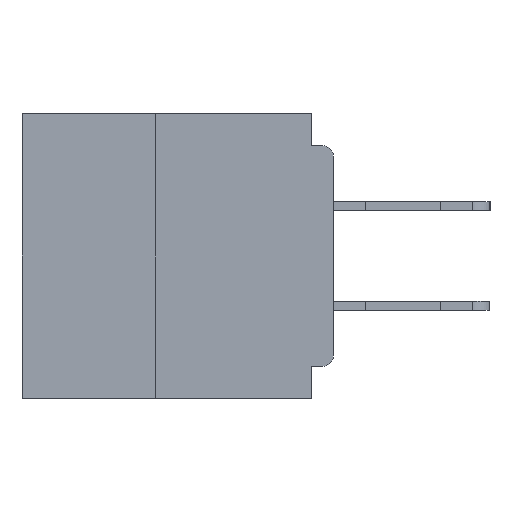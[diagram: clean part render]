
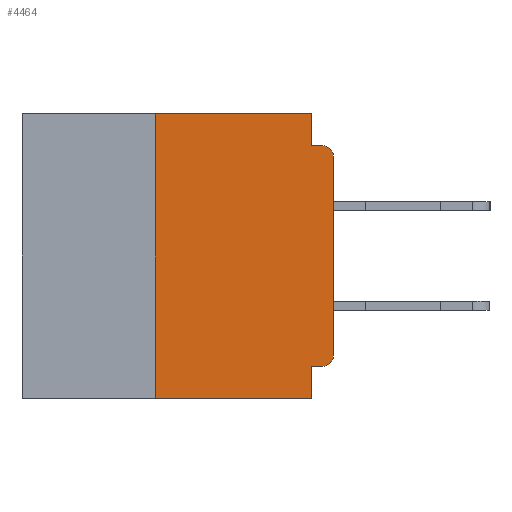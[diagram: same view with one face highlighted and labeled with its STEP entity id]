
A CAD part, left-side view. The second image highlights one B-rep face of the part: STEP entity #4464.
In plain terms, the highlighted planar face has unit normal (-1, 0, 0).
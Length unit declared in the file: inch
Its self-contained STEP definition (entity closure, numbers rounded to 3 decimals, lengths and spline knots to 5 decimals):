
#979 = CARTESIAN_POINT ( 'NONE',  ( 0., 0., 0. ) ) ;
#1393 = CIRCLE ( 'NONE', #21763, 0.015 ) ;
#1658 = EDGE_CURVE ( 'NONE', #28226, #30401, #25210, .T. ) ;
#2322 = DIRECTION ( 'NONE',  ( 0., 0., -1. ) ) ;
#2633 = VECTOR ( 'NONE', #27690, 39.37008 ) ;
#4018 = VERTEX_POINT ( 'NONE', #12158 ) ;
#4464 = ADVANCED_FACE ( 'NONE', ( #49938 ), #48460, .F. ) ;
#4643 = EDGE_CURVE ( 'NONE', #47357, #49684, #7635, .T. ) ;
#5485 = EDGE_CURVE ( 'NONE', #50651, #19949, #56696, .T. ) ;
#5751 = DIRECTION ( 'NONE',  ( 0., -1., 0. ) ) ;
#5847 = VECTOR ( 'NONE', #5751, 39.37008 ) ;
#5900 = CARTESIAN_POINT ( 'NONE',  ( 0., 0.015, -0.045 ) ) ;
#6881 = ORIENTED_EDGE ( 'NONE', *, *, #41117, .F. ) ;
#7635 = LINE ( 'NONE', #42677, #29825 ) ;
#7638 = VERTEX_POINT ( 'NONE', #51411 ) ;
#8385 = ORIENTED_EDGE ( 'NONE', *, *, #4643, .F. ) ;
#8566 = LINE ( 'NONE', #27789, #5847 ) ;
#9290 = CIRCLE ( 'NONE', #51377, 0.015 ) ;
#12158 = CARTESIAN_POINT ( 'NONE',  ( 0., 0., -0.34 ) ) ;
#12399 = EDGE_LOOP ( 'NONE', ( #20081, #30824, #6881, #8385, #30705, #33335, #28676, #15061, #35277, #37969 ) ) ;
#12461 = EDGE_CURVE ( 'NONE', #50651, #4018, #1393, .T. ) ;
#13020 = DIRECTION ( 'NONE',  ( -1., 0., 0. ) ) ;
#13493 = CARTESIAN_POINT ( 'NONE',  ( 0., 0.25, -0.4 ) ) ;
#14095 = VECTOR ( 'NONE', #56162, 39.37008 ) ;
#14364 = LINE ( 'NONE', #979, #2633 ) ;
#14510 = DIRECTION ( 'NONE',  ( 0., 1., 0. ) ) ;
#14691 = CARTESIAN_POINT ( 'NONE',  ( 0., 0., -0.355 ) ) ;
#15061 = ORIENTED_EDGE ( 'NONE', *, *, #35405, .F. ) ;
#17020 = AXIS2_PLACEMENT_3D ( 'NONE', #48537, #48074, #47954 ) ;
#19949 = VERTEX_POINT ( 'NONE', #34161 ) ;
#20081 = ORIENTED_EDGE ( 'NONE', *, *, #24008, .T. ) ;
#20784 = CARTESIAN_POINT ( 'NONE',  ( 0., 0.437, -0.4 ) ) ;
#21763 = AXIS2_PLACEMENT_3D ( 'NONE', #39619, #13020, #44067 ) ;
#23335 = CARTESIAN_POINT ( 'NONE',  ( 0., 0.437, 0. ) ) ;
#24008 = EDGE_CURVE ( 'NONE', #4018, #7638, #14364, .T. ) ;
#25210 = LINE ( 'NONE', #47474, #46081 ) ;
#25647 = CARTESIAN_POINT ( 'NONE',  ( 0., 0.031, -0.4 ) ) ;
#27124 = VERTEX_POINT ( 'NONE', #5900 ) ;
#27690 = DIRECTION ( 'NONE',  ( 0., 0., 1. ) ) ;
#27789 = CARTESIAN_POINT ( 'NONE',  ( 0., 0., -0.045 ) ) ;
#28226 = VERTEX_POINT ( 'NONE', #13493 ) ;
#28676 = ORIENTED_EDGE ( 'NONE', *, *, #41372, .T. ) ;
#28835 = DIRECTION ( 'NONE',  ( -1., 0., 0. ) ) ;
#29825 = VECTOR ( 'NONE', #42312, 39.37008 ) ;
#30401 = VERTEX_POINT ( 'NONE', #48843 ) ;
#30705 = ORIENTED_EDGE ( 'NONE', *, *, #34833, .F. ) ;
#30819 = CARTESIAN_POINT ( 'NONE',  ( 0., 0.015, -0.355 ) ) ;
#30824 = ORIENTED_EDGE ( 'NONE', *, *, #36242, .T. ) ;
#33204 = VECTOR ( 'NONE', #14510, 39.37008 ) ;
#33335 = ORIENTED_EDGE ( 'NONE', *, *, #1658, .F. ) ;
#34161 = CARTESIAN_POINT ( 'NONE',  ( 0., 0.031, -0.355 ) ) ;
#34353 = CARTESIAN_POINT ( 'NONE',  ( 0., 0.031, 0. ) ) ;
#34433 = VECTOR ( 'NONE', #45466, 39.37008 ) ;
#34833 = EDGE_CURVE ( 'NONE', #30401, #47357, #35826, .T. ) ;
#35277 = ORIENTED_EDGE ( 'NONE', *, *, #5485, .F. ) ;
#35405 = EDGE_CURVE ( 'NONE', #19949, #40076, #52358, .T. ) ;
#35826 = LINE ( 'NONE', #23335, #34433 ) ;
#36242 = EDGE_CURVE ( 'NONE', #7638, #27124, #9290, .T. ) ;
#37969 = ORIENTED_EDGE ( 'NONE', *, *, #12461, .T. ) ;
#39096 = LINE ( 'NONE', #20784, #14095 ) ;
#39619 = CARTESIAN_POINT ( 'NONE',  ( 0., 0.015, -0.34 ) ) ;
#40076 = VERTEX_POINT ( 'NONE', #25647 ) ;
#40158 = CARTESIAN_POINT ( 'NONE',  ( 0., 0.031, -0.4 ) ) ;
#40649 = VECTOR ( 'NONE', #53262, 39.37008 ) ;
#41117 = EDGE_CURVE ( 'NONE', #49684, #27124, #8566, .T. ) ;
#41372 = EDGE_CURVE ( 'NONE', #28226, #40076, #39096, .T. ) ;
#42312 = DIRECTION ( 'NONE',  ( 0., 0., -1. ) ) ;
#42677 = CARTESIAN_POINT ( 'NONE',  ( 0., 0.031, 0. ) ) ;
#44067 = DIRECTION ( 'NONE',  ( 0., 0., -1. ) ) ;
#45466 = DIRECTION ( 'NONE',  ( 0., -1., 0. ) ) ;
#46069 = CARTESIAN_POINT ( 'NONE',  ( 0., 0.031, -0.045 ) ) ;
#46081 = VECTOR ( 'NONE', #49469, 39.37008 ) ;
#47357 = VERTEX_POINT ( 'NONE', #34353 ) ;
#47474 = CARTESIAN_POINT ( 'NONE',  ( 0., 0.25, -0.4 ) ) ;
#47954 = DIRECTION ( 'NONE',  ( 0., 0., -1. ) ) ;
#48074 = DIRECTION ( 'NONE',  ( 1., 0., 0. ) ) ;
#48460 = PLANE ( 'NONE',  #17020 ) ;
#48537 = CARTESIAN_POINT ( 'NONE',  ( 0., 0.437, 0. ) ) ;
#48843 = CARTESIAN_POINT ( 'NONE',  ( 0., 0.25, 0. ) ) ;
#49469 = DIRECTION ( 'NONE',  ( 0., 0., 1. ) ) ;
#49684 = VERTEX_POINT ( 'NONE', #46069 ) ;
#49938 = FACE_OUTER_BOUND ( 'NONE', #12399, .T. ) ;
#50651 = VERTEX_POINT ( 'NONE', #30819 ) ;
#51377 = AXIS2_PLACEMENT_3D ( 'NONE', #55283, #28835, #2322 ) ;
#51411 = CARTESIAN_POINT ( 'NONE',  ( 0., 0., -0.06 ) ) ;
#52358 = LINE ( 'NONE', #40158, #40649 ) ;
#53262 = DIRECTION ( 'NONE',  ( 0., 0., -1. ) ) ;
#55283 = CARTESIAN_POINT ( 'NONE',  ( 0., 0.015, -0.06 ) ) ;
#56162 = DIRECTION ( 'NONE',  ( 0., -1., 0. ) ) ;
#56696 = LINE ( 'NONE', #14691, #33204 ) ;
